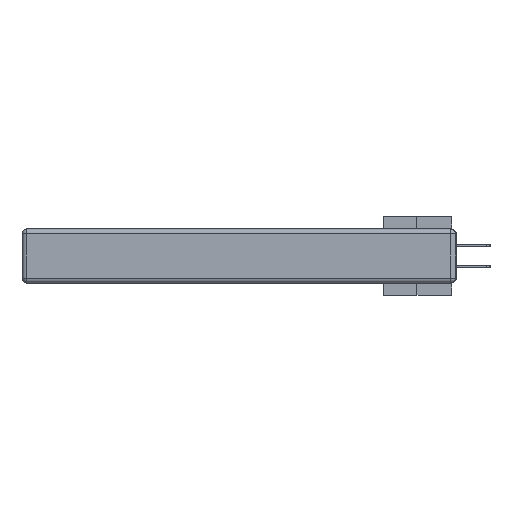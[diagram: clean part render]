
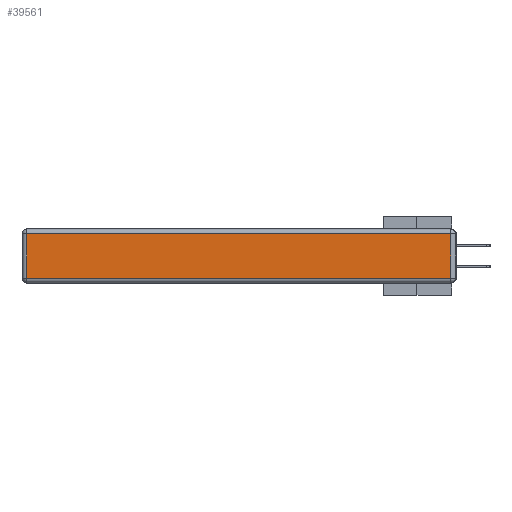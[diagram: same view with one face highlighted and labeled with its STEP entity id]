
A CAD part, left-side view. The second image highlights one B-rep face of the part: STEP entity #39561.
In plain terms, the highlighted planar face has unit normal (-1, 0, 0).
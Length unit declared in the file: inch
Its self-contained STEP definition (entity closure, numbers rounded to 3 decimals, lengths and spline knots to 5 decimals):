
#2165 = VECTOR ( 'NONE', #4738, 39.37008 ) ;
#2193 = CARTESIAN_POINT ( 'NONE',  ( 0., 0.03, -0.313 ) ) ;
#2322 = DIRECTION ( 'NONE',  ( 0., 1., 0. ) ) ;
#3240 = DIRECTION ( 'NONE',  ( -1., 0., 0. ) ) ;
#4738 = DIRECTION ( 'NONE',  ( 0., 0., 1. ) ) ;
#8880 = EDGE_LOOP ( 'NONE', ( #31040, #26087, #24702, #12043 ) ) ;
#11219 = DIRECTION ( 'NONE',  ( 0., -1., 0. ) ) ;
#12043 = ORIENTED_EDGE ( 'NONE', *, *, #32407, .T. ) ;
#12519 = VERTEX_POINT ( 'NONE', #29029 ) ;
#16601 = VERTEX_POINT ( 'NONE', #27767 ) ;
#16830 = CARTESIAN_POINT ( 'NONE',  ( 0., 0., -0.343 ) ) ;
#18327 = VECTOR ( 'NONE', #11219, 39.37008 ) ;
#18857 = VECTOR ( 'NONE', #43615, 39.37008 ) ;
#21000 = CARTESIAN_POINT ( 'NONE',  ( 0., 2.72, -0.313 ) ) ;
#24702 = ORIENTED_EDGE ( 'NONE', *, *, #27794, .T. ) ;
#26087 = ORIENTED_EDGE ( 'NONE', *, *, #30003, .T. ) ;
#27767 = CARTESIAN_POINT ( 'NONE',  ( 0., 2.72, -0.03 ) ) ;
#27794 = EDGE_CURVE ( 'NONE', #12519, #16601, #34431, .T. ) ;
#28062 = CARTESIAN_POINT ( 'NONE',  ( 0., 0., -0.313 ) ) ;
#29029 = CARTESIAN_POINT ( 'NONE',  ( 0., 0.03, -0.03 ) ) ;
#29279 = EDGE_CURVE ( 'NONE', #43411, #39324, #34307, .T. ) ;
#29313 = CARTESIAN_POINT ( 'NONE',  ( 0., 2.75, -0.03 ) ) ;
#30003 = EDGE_CURVE ( 'NONE', #39324, #12519, #31017, .T. ) ;
#31017 = LINE ( 'NONE', #38760, #2165 ) ;
#31040 = ORIENTED_EDGE ( 'NONE', *, *, #29279, .T. ) ;
#32407 = EDGE_CURVE ( 'NONE', #16601, #43411, #39650, .T. ) ;
#32437 = AXIS2_PLACEMENT_3D ( 'NONE', #16830, #3240, #40702 ) ;
#34307 = LINE ( 'NONE', #28062, #18327 ) ;
#34431 = LINE ( 'NONE', #29313, #40865 ) ;
#37276 = PLANE ( 'NONE',  #32437 ) ;
#38588 = FACE_OUTER_BOUND ( 'NONE', #8880, .T. ) ;
#38760 = CARTESIAN_POINT ( 'NONE',  ( 0., 0.03, -0.343 ) ) ;
#39324 = VERTEX_POINT ( 'NONE', #2193 ) ;
#39561 = ADVANCED_FACE ( 'NONE', ( #38588 ), #37276, .T. ) ;
#39650 = LINE ( 'NONE', #40180, #18857 ) ;
#40180 = CARTESIAN_POINT ( 'NONE',  ( 0., 2.72, -0.343 ) ) ;
#40702 = DIRECTION ( 'NONE',  ( 0., 0., 1. ) ) ;
#40865 = VECTOR ( 'NONE', #2322, 39.37008 ) ;
#43411 = VERTEX_POINT ( 'NONE', #21000 ) ;
#43615 = DIRECTION ( 'NONE',  ( 0., 0., -1. ) ) ;
